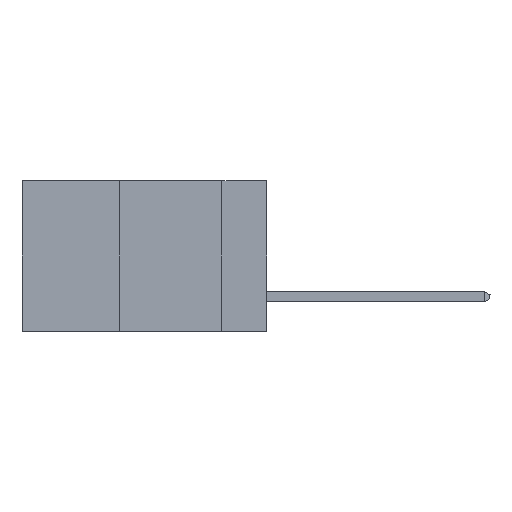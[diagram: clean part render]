
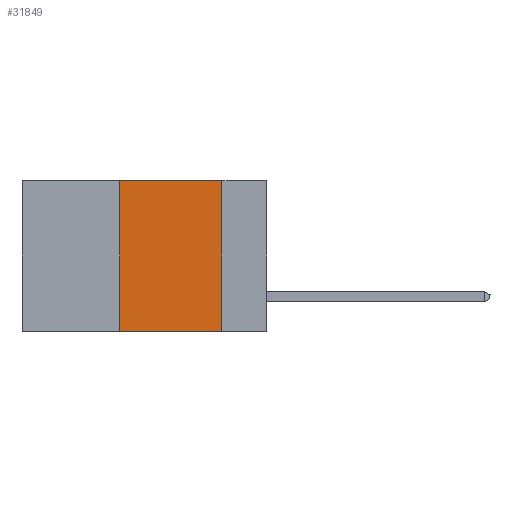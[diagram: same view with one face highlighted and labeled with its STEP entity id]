
A CAD part, left-side view. The second image highlights one B-rep face of the part: STEP entity #31849.
In plain terms, the highlighted planar face has unit normal (-1, 0, 0).
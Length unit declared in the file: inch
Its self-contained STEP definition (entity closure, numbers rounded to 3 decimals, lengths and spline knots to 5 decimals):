
#2028 = EDGE_CURVE ( 'NONE', #24621, #43326, #30442, .T. ) ;
#2066 = LINE ( 'NONE', #30634, #8029 ) ;
#2146 = ORIENTED_EDGE ( 'NONE', *, *, #39659, .F. ) ;
#2412 = CARTESIAN_POINT ( 'NONE',  ( 0., 0.6, -0.37 ) ) ;
#3534 = PLANE ( 'NONE',  #6695 ) ;
#5923 = DIRECTION ( 'NONE',  ( 0., -1., 0. ) ) ;
#6695 = AXIS2_PLACEMENT_3D ( 'NONE', #7015, #41561, #24335 ) ;
#7015 = CARTESIAN_POINT ( 'NONE',  ( 0., 0.6, 0. ) ) ;
#7441 = LINE ( 'NONE', #2412, #24168 ) ;
#8029 = VECTOR ( 'NONE', #34089, 39.37008 ) ;
#8135 = LINE ( 'NONE', #11003, #34557 ) ;
#8964 = CARTESIAN_POINT ( 'NONE',  ( 0., 0.36, 0. ) ) ;
#9516 = EDGE_LOOP ( 'NONE', ( #34355, #2146, #36557, #24803 ) ) ;
#10026 = DIRECTION ( 'NONE',  ( 0., 0., 1. ) ) ;
#10833 = CARTESIAN_POINT ( 'NONE',  ( 0., 0.11, -0.37 ) ) ;
#11003 = CARTESIAN_POINT ( 'NONE',  ( 0., 0.11, 0. ) ) ;
#12317 = VERTEX_POINT ( 'NONE', #31843 ) ;
#15006 = FACE_OUTER_BOUND ( 'NONE', #9516, .T. ) ;
#16174 = EDGE_CURVE ( 'NONE', #24621, #24240, #7441, .T. ) ;
#22701 = CARTESIAN_POINT ( 'NONE',  ( 0., 0.36, -0.37 ) ) ;
#24168 = VECTOR ( 'NONE', #5923, 39.37008 ) ;
#24240 = VERTEX_POINT ( 'NONE', #10833 ) ;
#24335 = DIRECTION ( 'NONE',  ( 0., 0., -1. ) ) ;
#24621 = VERTEX_POINT ( 'NONE', #22701 ) ;
#24803 = ORIENTED_EDGE ( 'NONE', *, *, #16174, .T. ) ;
#28364 = DIRECTION ( 'NONE',  ( 0., 0., -1. ) ) ;
#29348 = VECTOR ( 'NONE', #10026, 39.37008 ) ;
#30442 = LINE ( 'NONE', #38093, #29348 ) ;
#30634 = CARTESIAN_POINT ( 'NONE',  ( 0., 0.6, 0. ) ) ;
#31843 = CARTESIAN_POINT ( 'NONE',  ( 0., 0.11, 0. ) ) ;
#31849 = ADVANCED_FACE ( 'NONE', ( #15006 ), #3534, .F. ) ;
#34089 = DIRECTION ( 'NONE',  ( 0., -1., 0. ) ) ;
#34355 = ORIENTED_EDGE ( 'NONE', *, *, #43764, .F. ) ;
#34557 = VECTOR ( 'NONE', #28364, 39.37008 ) ;
#36557 = ORIENTED_EDGE ( 'NONE', *, *, #2028, .F. ) ;
#38093 = CARTESIAN_POINT ( 'NONE',  ( 0., 0.36, 0. ) ) ;
#39659 = EDGE_CURVE ( 'NONE', #43326, #12317, #2066, .T. ) ;
#41561 = DIRECTION ( 'NONE',  ( 1., 0., 0. ) ) ;
#43326 = VERTEX_POINT ( 'NONE', #8964 ) ;
#43764 = EDGE_CURVE ( 'NONE', #12317, #24240, #8135, .T. ) ;
